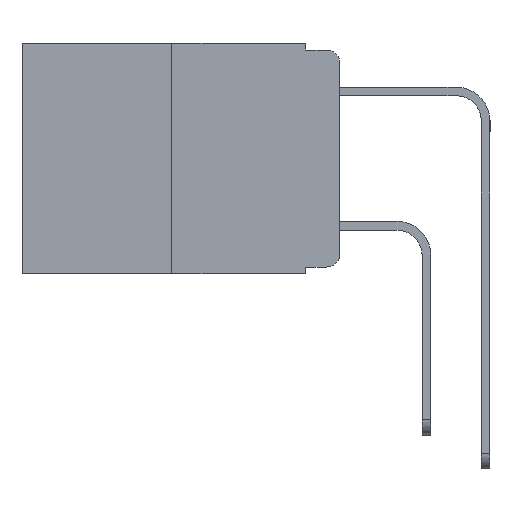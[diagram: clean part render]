
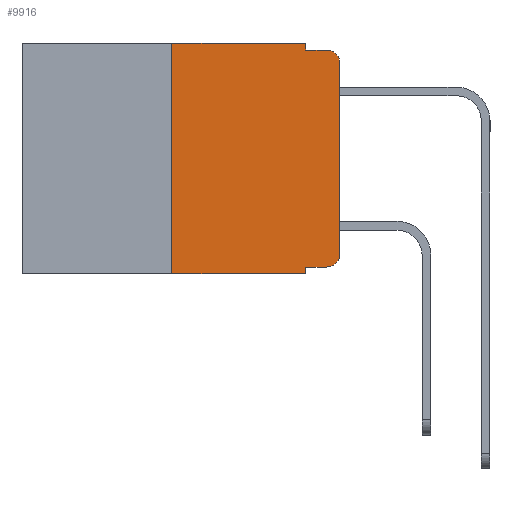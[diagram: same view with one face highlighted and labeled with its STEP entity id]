
A CAD part, left-side view. The second image highlights one B-rep face of the part: STEP entity #9916.
In plain terms, the highlighted planar face has unit normal (-1, 0, 0).
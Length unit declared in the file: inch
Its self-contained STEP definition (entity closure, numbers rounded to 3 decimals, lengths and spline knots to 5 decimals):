
#280 = CARTESIAN_POINT ( 'NONE',  ( 0., 0.02, -0.313 ) ) ;
#391 = CARTESIAN_POINT ( 'NONE',  ( 0., 0.051, -0.01 ) ) ;
#488 = EDGE_CURVE ( 'NONE', #10733, #7173, #6867, .T. ) ;
#600 = EDGE_CURVE ( 'NONE', #15194, #7173, #15499, .T. ) ;
#838 = ORIENTED_EDGE ( 'NONE', *, *, #600, .T. ) ;
#933 = LINE ( 'NONE', #8605, #10518 ) ;
#1713 = DIRECTION ( 'NONE',  ( 0., 0., -1. ) ) ;
#1729 = VECTOR ( 'NONE', #7276, 39.37008 ) ;
#1908 = CIRCLE ( 'NONE', #4794, 0.02 ) ;
#2170 = CARTESIAN_POINT ( 'NONE',  ( 0., 0., -0.03 ) ) ;
#2174 = FACE_OUTER_BOUND ( 'NONE', #6648, .T. ) ;
#2434 = CARTESIAN_POINT ( 'NONE',  ( 0., 0.25, 0. ) ) ;
#2629 = DIRECTION ( 'NONE',  ( 0., 0., -1. ) ) ;
#2688 = CARTESIAN_POINT ( 'NONE',  ( 0., 0.473, -0.343 ) ) ;
#2891 = CARTESIAN_POINT ( 'NONE',  ( 0., 0., 0. ) ) ;
#2895 = CARTESIAN_POINT ( 'NONE',  ( 0., 0.051, 0. ) ) ;
#3591 = CARTESIAN_POINT ( 'NONE',  ( 0., 0.051, -0.333 ) ) ;
#3837 = DIRECTION ( 'NONE',  ( 0., 0., -1. ) ) ;
#3910 = EDGE_CURVE ( 'NONE', #4039, #6672, #11821, .T. ) ;
#3949 = EDGE_CURVE ( 'NONE', #14793, #9220, #11012, .T. ) ;
#4039 = VERTEX_POINT ( 'NONE', #14422 ) ;
#4193 = CARTESIAN_POINT ( 'NONE',  ( 0., 0.051, 0. ) ) ;
#4298 = CARTESIAN_POINT ( 'NONE',  ( 0., 0.25, -0.343 ) ) ;
#4347 = DIRECTION ( 'NONE',  ( 1., 0., 0. ) ) ;
#4349 = ORIENTED_EDGE ( 'NONE', *, *, #488, .F. ) ;
#4782 = CARTESIAN_POINT ( 'NONE',  ( 0., 0.02, -0.333 ) ) ;
#4794 = AXIS2_PLACEMENT_3D ( 'NONE', #280, #9492, #1713 ) ;
#4795 = VECTOR ( 'NONE', #13203, 39.37008 ) ;
#4867 = DIRECTION ( 'NONE',  ( 0., 0., -1. ) ) ;
#4887 = DIRECTION ( 'NONE',  ( -1., 0., 0. ) ) ;
#4948 = VECTOR ( 'NONE', #3837, 39.37008 ) ;
#5335 = CARTESIAN_POINT ( 'NONE',  ( 0., 0.02, -0.03 ) ) ;
#5641 = PLANE ( 'NONE',  #10823 ) ;
#5693 = CARTESIAN_POINT ( 'NONE',  ( 0., 0.051, -0.343 ) ) ;
#5816 = ORIENTED_EDGE ( 'NONE', *, *, #3949, .T. ) ;
#5939 = LINE ( 'NONE', #12332, #15813 ) ;
#6147 = EDGE_CURVE ( 'NONE', #11708, #4039, #5939, .T. ) ;
#6258 = VERTEX_POINT ( 'NONE', #4782 ) ;
#6648 = EDGE_LOOP ( 'NONE', ( #12273, #5816, #9235, #13079, #16504, #13891, #838, #4349, #7832, #14697 ) ) ;
#6672 = VERTEX_POINT ( 'NONE', #391 ) ;
#6867 = LINE ( 'NONE', #2895, #16721 ) ;
#7173 = VERTEX_POINT ( 'NONE', #5693 ) ;
#7207 = DIRECTION ( 'NONE',  ( 0., -1., 0. ) ) ;
#7276 = DIRECTION ( 'NONE',  ( 0., -1., 0. ) ) ;
#7832 = ORIENTED_EDGE ( 'NONE', *, *, #16224, .T. ) ;
#7970 = VERTEX_POINT ( 'NONE', #15019 ) ;
#7983 = EDGE_CURVE ( 'NONE', #15194, #11708, #933, .T. ) ;
#8605 = CARTESIAN_POINT ( 'NONE',  ( 0., 0.25, 0. ) ) ;
#8704 = AXIS2_PLACEMENT_3D ( 'NONE', #5335, #4887, #4867 ) ;
#9220 = VERTEX_POINT ( 'NONE', #14577 ) ;
#9235 = ORIENTED_EDGE ( 'NONE', *, *, #10367, .F. ) ;
#9492 = DIRECTION ( 'NONE',  ( -1., 0., 0. ) ) ;
#9916 = ADVANCED_FACE ( 'NONE', ( #2174 ), #5641, .F. ) ;
#10367 = EDGE_CURVE ( 'NONE', #6672, #9220, #15115, .T. ) ;
#10373 = VECTOR ( 'NONE', #14579, 39.37008 ) ;
#10518 = VECTOR ( 'NONE', #12394, 39.37008 ) ;
#10733 = VERTEX_POINT ( 'NONE', #3591 ) ;
#10823 = AXIS2_PLACEMENT_3D ( 'NONE', #12134, #4347, #13436 ) ;
#11012 = CIRCLE ( 'NONE', #8704, 0.02 ) ;
#11632 = CARTESIAN_POINT ( 'NONE',  ( 0., 0.051, -0.333 ) ) ;
#11708 = VERTEX_POINT ( 'NONE', #2434 ) ;
#11821 = LINE ( 'NONE', #4193, #4948 ) ;
#12134 = CARTESIAN_POINT ( 'NONE',  ( 0., 0.473, 0. ) ) ;
#12273 = ORIENTED_EDGE ( 'NONE', *, *, #16392, .T. ) ;
#12332 = CARTESIAN_POINT ( 'NONE',  ( 0., 0.473, 0. ) ) ;
#12394 = DIRECTION ( 'NONE',  ( 0., 0., 1. ) ) ;
#13079 = ORIENTED_EDGE ( 'NONE', *, *, #3910, .F. ) ;
#13203 = DIRECTION ( 'NONE',  ( 0., -1., 0. ) ) ;
#13436 = DIRECTION ( 'NONE',  ( 0., 0., -1. ) ) ;
#13837 = LINE ( 'NONE', #2891, #10373 ) ;
#13891 = ORIENTED_EDGE ( 'NONE', *, *, #7983, .F. ) ;
#14422 = CARTESIAN_POINT ( 'NONE',  ( 0., 0.051, 0. ) ) ;
#14550 = EDGE_CURVE ( 'NONE', #6258, #7970, #1908, .T. ) ;
#14577 = CARTESIAN_POINT ( 'NONE',  ( 0., 0.02, -0.01 ) ) ;
#14579 = DIRECTION ( 'NONE',  ( 0., 0., 1. ) ) ;
#14697 = ORIENTED_EDGE ( 'NONE', *, *, #14550, .T. ) ;
#14793 = VERTEX_POINT ( 'NONE', #2170 ) ;
#15019 = CARTESIAN_POINT ( 'NONE',  ( 0., 0., -0.313 ) ) ;
#15115 = LINE ( 'NONE', #15763, #4795 ) ;
#15194 = VERTEX_POINT ( 'NONE', #4298 ) ;
#15499 = LINE ( 'NONE', #2688, #1729 ) ;
#15523 = DIRECTION ( 'NONE',  ( 0., -1., 0. ) ) ;
#15763 = CARTESIAN_POINT ( 'NONE',  ( 0., 0.051, -0.01 ) ) ;
#15813 = VECTOR ( 'NONE', #7207, 39.37008 ) ;
#16224 = EDGE_CURVE ( 'NONE', #10733, #6258, #16659, .T. ) ;
#16254 = VECTOR ( 'NONE', #15523, 39.37008 ) ;
#16392 = EDGE_CURVE ( 'NONE', #7970, #14793, #13837, .T. ) ;
#16504 = ORIENTED_EDGE ( 'NONE', *, *, #6147, .F. ) ;
#16659 = LINE ( 'NONE', #11632, #16254 ) ;
#16721 = VECTOR ( 'NONE', #2629, 39.37008 ) ;
